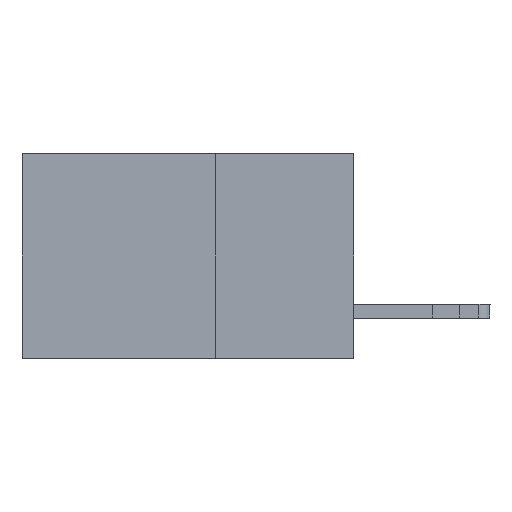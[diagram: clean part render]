
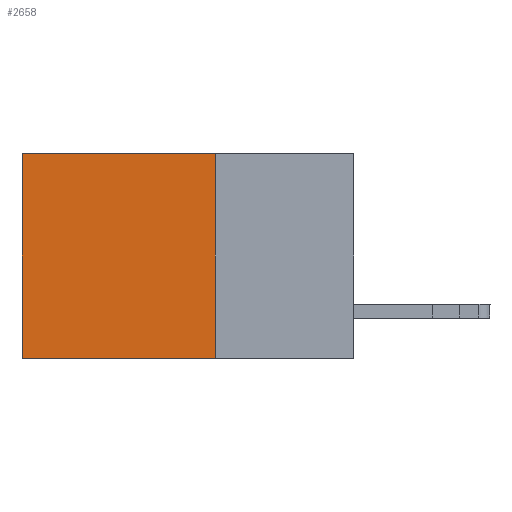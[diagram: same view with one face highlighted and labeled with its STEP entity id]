
A CAD part, left-side view. The second image highlights one B-rep face of the part: STEP entity #2658.
In plain terms, the highlighted planar face has unit normal (-1, 0, 0).
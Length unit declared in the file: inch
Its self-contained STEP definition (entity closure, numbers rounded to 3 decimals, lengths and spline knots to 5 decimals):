
#299 = DIRECTION ( 'NONE',  ( 0., 0., -1. ) ) ;
#629 = CARTESIAN_POINT ( 'NONE',  ( 0.2875, 0.6, -0.37 ) ) ;
#718 = VECTOR ( 'NONE', #12258, 39.37008 ) ;
#753 = CARTESIAN_POINT ( 'NONE',  ( 0.2875, 0.25, 0. ) ) ;
#2304 = PLANE ( 'NONE',  #9844 ) ;
#2658 = ADVANCED_FACE ( 'NONE', ( #11983 ), #2304, .F. ) ;
#2690 = CARTESIAN_POINT ( 'NONE',  ( 0.2875, 0.6, 0. ) ) ;
#2837 = EDGE_CURVE ( 'NONE', #16414, #6357, #17312, .T. ) ;
#3159 = VERTEX_POINT ( 'NONE', #8788 ) ;
#3394 = LINE ( 'NONE', #6034, #4039 ) ;
#3901 = CARTESIAN_POINT ( 'NONE',  ( 0.2875, 0.25, 0. ) ) ;
#4039 = VECTOR ( 'NONE', #299, 39.37008 ) ;
#4114 = ORIENTED_EDGE ( 'NONE', *, *, #15764, .T. ) ;
#4551 = LINE ( 'NONE', #15282, #718 ) ;
#4610 = VECTOR ( 'NONE', #6776, 39.37008 ) ;
#6034 = CARTESIAN_POINT ( 'NONE',  ( 0.2875, 0.25, 0. ) ) ;
#6314 = ORIENTED_EDGE ( 'NONE', *, *, #14401, .F. ) ;
#6357 = VERTEX_POINT ( 'NONE', #17017 ) ;
#6768 = EDGE_CURVE ( 'NONE', #16414, #3159, #3394, .T. ) ;
#6776 = DIRECTION ( 'NONE',  ( 0., 1., 0. ) ) ;
#7031 = ORIENTED_EDGE ( 'NONE', *, *, #2837, .T. ) ;
#7904 = EDGE_LOOP ( 'NONE', ( #4114, #6314, #9978, #7031 ) ) ;
#8788 = CARTESIAN_POINT ( 'NONE',  ( 0.2875, 0.25, -0.37 ) ) ;
#9844 = AXIS2_PLACEMENT_3D ( 'NONE', #753, #15059, #10742 ) ;
#9978 = ORIENTED_EDGE ( 'NONE', *, *, #6768, .F. ) ;
#10742 = DIRECTION ( 'NONE',  ( 0., 0., -1. ) ) ;
#11372 = DIRECTION ( 'NONE',  ( 0., 0., -1. ) ) ;
#11922 = LINE ( 'NONE', #2690, #12141 ) ;
#11983 = FACE_OUTER_BOUND ( 'NONE', #7904, .T. ) ;
#12141 = VECTOR ( 'NONE', #11372, 39.37008 ) ;
#12258 = DIRECTION ( 'NONE',  ( 0., 1., 0. ) ) ;
#12805 = CARTESIAN_POINT ( 'NONE',  ( 0.2875, 0.25, 0. ) ) ;
#14401 = EDGE_CURVE ( 'NONE', #3159, #18137, #4551, .T. ) ;
#15059 = DIRECTION ( 'NONE',  ( 1., 0., 0. ) ) ;
#15282 = CARTESIAN_POINT ( 'NONE',  ( 0.2875, 0.25, -0.37 ) ) ;
#15764 = EDGE_CURVE ( 'NONE', #6357, #18137, #11922, .T. ) ;
#16414 = VERTEX_POINT ( 'NONE', #12805 ) ;
#17017 = CARTESIAN_POINT ( 'NONE',  ( 0.2875, 0.6, 0. ) ) ;
#17312 = LINE ( 'NONE', #3901, #4610 ) ;
#18137 = VERTEX_POINT ( 'NONE', #629 ) ;
